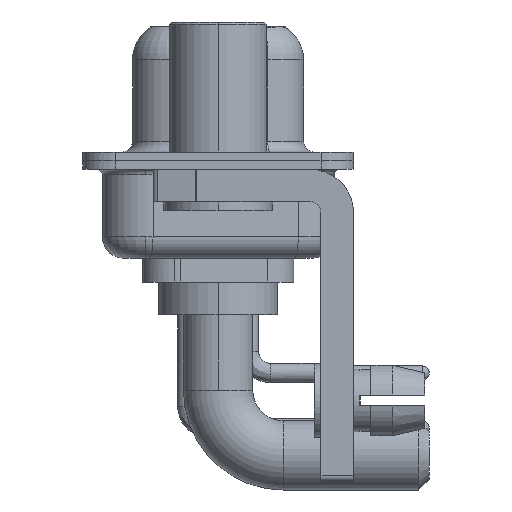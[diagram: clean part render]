
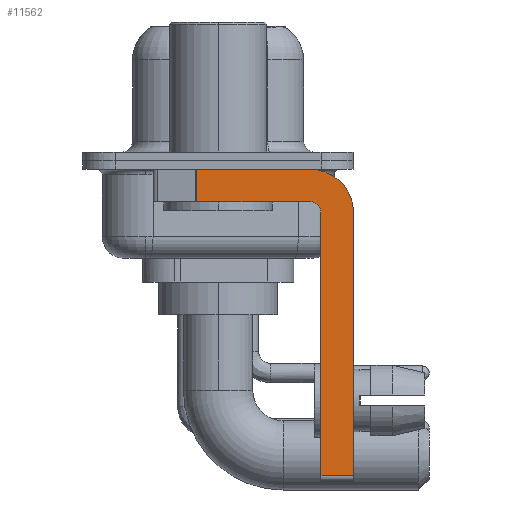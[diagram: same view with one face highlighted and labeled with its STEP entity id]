
A CAD part, left-side view. The second image highlights one B-rep face of the part: STEP entity #11562.
In plain terms, the highlighted planar face has unit normal (-1, 0, 0).
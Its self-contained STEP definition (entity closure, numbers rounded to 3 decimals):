
#122 = AXIS2_PLACEMENT_3D ( 'NONE', #3262, #8536, #4867 ) ;
#515 = ORIENTED_EDGE ( 'NONE', *, *, #11911, .F. ) ;
#615 = LINE ( 'NONE', #7573, #21932 ) ;
#1094 = LINE ( 'NONE', #8291, #17534 ) ;
#1999 = LINE ( 'NONE', #18899, #20981 ) ;
#2855 = EDGE_CURVE ( 'NONE', #10207, #12698, #8357, .T. ) ;
#3165 = DIRECTION ( 'NONE',  ( 0., 0., 1. ) ) ;
#3262 = CARTESIAN_POINT ( 'NONE',  ( -2.9, -4.25, -2.4 ) ) ;
#3778 = CARTESIAN_POINT ( 'NONE',  ( -2.9, -6.25, -2.4 ) ) ;
#4138 = ORIENTED_EDGE ( 'NONE', *, *, #8731, .F. ) ;
#4357 = ORIENTED_EDGE ( 'NONE', *, *, #6666, .F. ) ;
#4588 = CARTESIAN_POINT ( 'NONE',  ( -2.9, -4.25, -1.9 ) ) ;
#4867 = DIRECTION ( 'NONE',  ( 0., 0., -1. ) ) ;
#4898 = AXIS2_PLACEMENT_3D ( 'NONE', #11049, #14572, #11159 ) ;
#5061 = EDGE_CURVE ( 'NONE', #7287, #20864, #8624, .T. ) ;
#5657 = VECTOR ( 'NONE', #13807, 1000. ) ;
#6343 = CARTESIAN_POINT ( 'NONE',  ( -2.9, 0.978, -1.9 ) ) ;
#6563 = LINE ( 'NONE', #6343, #21931 ) ;
#6666 = EDGE_CURVE ( 'NONE', #9381, #20864, #615, .T. ) ;
#7044 = LINE ( 'NONE', #20890, #5657 ) ;
#7287 = VERTEX_POINT ( 'NONE', #7566 ) ;
#7566 = CARTESIAN_POINT ( 'NONE',  ( -2.9, -4.75, -14.55 ) ) ;
#7573 = CARTESIAN_POINT ( 'NONE',  ( -2.9, -6.25, -2.4 ) ) ;
#8291 = CARTESIAN_POINT ( 'NONE',  ( -2.9, -4.75, -14.8 ) ) ;
#8357 = CIRCLE ( 'NONE', #10543, 0.5 ) ;
#8405 = CARTESIAN_POINT ( 'NONE',  ( -2.9, -4.25, -0.4 ) ) ;
#8506 = CARTESIAN_POINT ( 'NONE',  ( -2.9, -4.25, -14.55 ) ) ;
#8536 = DIRECTION ( 'NONE',  ( 1., 0., 0. ) ) ;
#8624 = LINE ( 'NONE', #8506, #12436 ) ;
#8731 = EDGE_CURVE ( 'NONE', #13165, #9381, #13986, .T. ) ;
#9228 = ORIENTED_EDGE ( 'NONE', *, *, #16741, .F. ) ;
#9276 = CARTESIAN_POINT ( 'NONE',  ( -2.9, 0.978, -1.9 ) ) ;
#9381 = VERTEX_POINT ( 'NONE', #3778 ) ;
#9792 = CARTESIAN_POINT ( 'NONE',  ( -2.9, -4.25, -2.4 ) ) ;
#10207 = VERTEX_POINT ( 'NONE', #16538 ) ;
#10543 = AXIS2_PLACEMENT_3D ( 'NONE', #9792, #22142, #3165 ) ;
#11049 = CARTESIAN_POINT ( 'NONE',  ( -2.9, -4.25, -2.4 ) ) ;
#11159 = DIRECTION ( 'NONE',  ( 0., 0., -1. ) ) ;
#11562 = ADVANCED_FACE ( 'NONE', ( #18116 ), #12874, .F. ) ;
#11911 = EDGE_CURVE ( 'NONE', #12698, #15620, #1999, .T. ) ;
#12153 = DIRECTION ( 'NONE',  ( 0., -1., 0. ) ) ;
#12436 = VECTOR ( 'NONE', #12153, 1000. ) ;
#12698 = VERTEX_POINT ( 'NONE', #4588 ) ;
#12874 = PLANE ( 'NONE',  #4898 ) ;
#12996 = VERTEX_POINT ( 'NONE', #14579 ) ;
#13165 = VERTEX_POINT ( 'NONE', #8405 ) ;
#13807 = DIRECTION ( 'NONE',  ( 0., -1., 0. ) ) ;
#13986 = CIRCLE ( 'NONE', #122, 2. ) ;
#14432 = DIRECTION ( 'NONE',  ( 0., 0., -1. ) ) ;
#14572 = DIRECTION ( 'NONE',  ( 1., 0., 0. ) ) ;
#14579 = CARTESIAN_POINT ( 'NONE',  ( -2.9, 0.978, -0.4 ) ) ;
#15281 = CARTESIAN_POINT ( 'NONE',  ( -2.9, -6.25, -14.55 ) ) ;
#15620 = VERTEX_POINT ( 'NONE', #9276 ) ;
#16538 = CARTESIAN_POINT ( 'NONE',  ( -2.9, -4.75, -2.4 ) ) ;
#16741 = EDGE_CURVE ( 'NONE', #7287, #10207, #1094, .T. ) ;
#16849 = EDGE_CURVE ( 'NONE', #12996, #15620, #6563, .T. ) ;
#17068 = ORIENTED_EDGE ( 'NONE', *, *, #2855, .F. ) ;
#17292 = DIRECTION ( 'NONE',  ( 0., 1., 0. ) ) ;
#17438 = EDGE_LOOP ( 'NONE', ( #20903, #22494, #515, #17068, #9228, #22212, #4357, #4138 ) ) ;
#17534 = VECTOR ( 'NONE', #22121, 1000. ) ;
#18116 = FACE_OUTER_BOUND ( 'NONE', #17438, .T. ) ;
#18899 = CARTESIAN_POINT ( 'NONE',  ( -2.9, -4.25, -1.9 ) ) ;
#18904 = DIRECTION ( 'NONE',  ( 0., 0., -1. ) ) ;
#20864 = VERTEX_POINT ( 'NONE', #15281 ) ;
#20890 = CARTESIAN_POINT ( 'NONE',  ( -2.9, 3., -0.4 ) ) ;
#20903 = ORIENTED_EDGE ( 'NONE', *, *, #22155, .F. ) ;
#20981 = VECTOR ( 'NONE', #17292, 1000. ) ;
#21931 = VECTOR ( 'NONE', #18904, 1000. ) ;
#21932 = VECTOR ( 'NONE', #14432, 1000. ) ;
#22121 = DIRECTION ( 'NONE',  ( 0., 0., 1. ) ) ;
#22142 = DIRECTION ( 'NONE',  ( -1., 0., 0. ) ) ;
#22155 = EDGE_CURVE ( 'NONE', #12996, #13165, #7044, .T. ) ;
#22212 = ORIENTED_EDGE ( 'NONE', *, *, #5061, .T. ) ;
#22494 = ORIENTED_EDGE ( 'NONE', *, *, #16849, .T. ) ;
